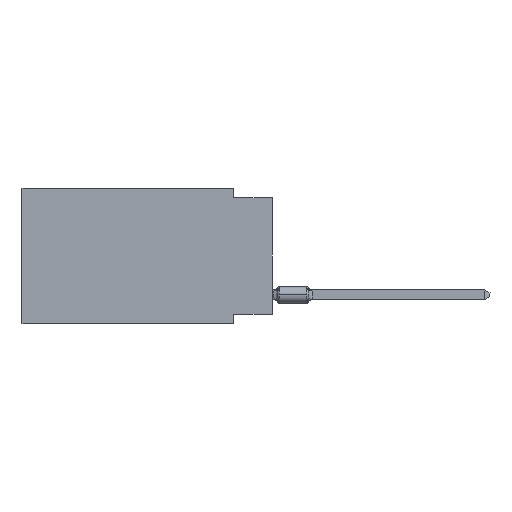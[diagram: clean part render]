
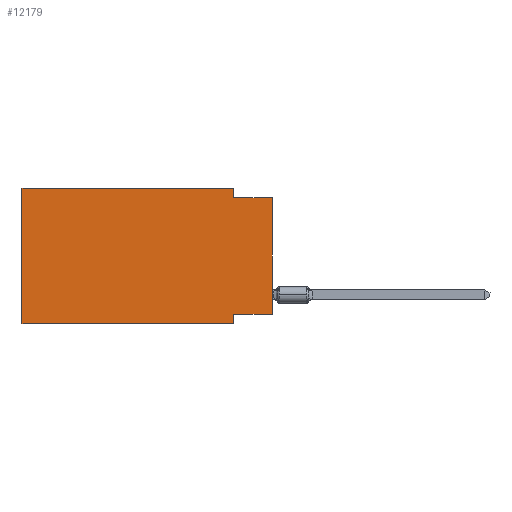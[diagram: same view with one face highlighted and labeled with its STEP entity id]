
A CAD part, left-side view. The second image highlights one B-rep face of the part: STEP entity #12179.
In plain terms, the highlighted planar face has unit normal (-1, 0, 0).
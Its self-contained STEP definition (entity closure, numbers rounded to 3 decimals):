
#191 = DIRECTION ( 'NONE',  ( 0., -1., 0. ) ) ;
#363 = EDGE_CURVE ( 'NONE', #18835, #9206, #13381, .T. ) ;
#1158 = VECTOR ( 'NONE', #7024, 1000. ) ;
#1394 = PLANE ( 'NONE',  #21384 ) ;
#1685 = DIRECTION ( 'NONE',  ( 0., 0., 1. ) ) ;
#1731 = CARTESIAN_POINT ( 'NONE',  ( 0., 0., -8.255 ) ) ;
#1751 = VECTOR ( 'NONE', #11459, 1000. ) ;
#1968 = DIRECTION ( 'NONE',  ( 0., 0., -1. ) ) ;
#2621 = ORIENTED_EDGE ( 'NONE', *, *, #363, .T. ) ;
#2857 = ORIENTED_EDGE ( 'NONE', *, *, #15554, .F. ) ;
#3054 = CARTESIAN_POINT ( 'NONE',  ( 0., 2.54, -8.89 ) ) ;
#4588 = EDGE_CURVE ( 'NONE', #18835, #18418, #22463, .T. ) ;
#4745 = CARTESIAN_POINT ( 'NONE',  ( 0., 16.383, -8.89 ) ) ;
#4921 = CARTESIAN_POINT ( 'NONE',  ( 0., 2.54, 0. ) ) ;
#6089 = VECTOR ( 'NONE', #29303, 1000. ) ;
#6251 = ORIENTED_EDGE ( 'NONE', *, *, #4588, .F. ) ;
#7024 = DIRECTION ( 'NONE',  ( 0., -1., 0. ) ) ;
#7233 = ORIENTED_EDGE ( 'NONE', *, *, #13359, .F. ) ;
#7501 = EDGE_CURVE ( 'NONE', #17132, #9206, #8265, .T. ) ;
#7999 = CARTESIAN_POINT ( 'NONE',  ( 0., 16.383, -8.89 ) ) ;
#8095 = CARTESIAN_POINT ( 'NONE',  ( 0., 0., -8.255 ) ) ;
#8265 = LINE ( 'NONE', #15932, #18362 ) ;
#8808 = EDGE_CURVE ( 'NONE', #25202, #20504, #13998, .T. ) ;
#9206 = VERTEX_POINT ( 'NONE', #28959 ) ;
#9609 = LINE ( 'NONE', #27790, #28229 ) ;
#11302 = ORIENTED_EDGE ( 'NONE', *, *, #7501, .F. ) ;
#11459 = DIRECTION ( 'NONE',  ( 0., 0., -1. ) ) ;
#12179 = ADVANCED_FACE ( 'NONE', ( #21865 ), #1394, .F. ) ;
#12879 = VECTOR ( 'NONE', #26718, 1000. ) ;
#13359 = EDGE_CURVE ( 'NONE', #18418, #23145, #26578, .T. ) ;
#13381 = LINE ( 'NONE', #24738, #22741 ) ;
#13714 = LINE ( 'NONE', #4745, #1158 ) ;
#13998 = LINE ( 'NONE', #23222, #14614 ) ;
#14471 = ORIENTED_EDGE ( 'NONE', *, *, #8808, .F. ) ;
#14550 = VERTEX_POINT ( 'NONE', #21872 ) ;
#14614 = VECTOR ( 'NONE', #27935, 1000. ) ;
#15401 = ORIENTED_EDGE ( 'NONE', *, *, #26850, .F. ) ;
#15554 = EDGE_CURVE ( 'NONE', #14550, #17132, #22824, .T. ) ;
#15932 = CARTESIAN_POINT ( 'NONE',  ( 0., 0., -0.635 ) ) ;
#17024 = CARTESIAN_POINT ( 'NONE',  ( 0., 2.54, -8.89 ) ) ;
#17132 = VERTEX_POINT ( 'NONE', #23230 ) ;
#17757 = DIRECTION ( 'NONE',  ( 1., 0., 0. ) ) ;
#18362 = VECTOR ( 'NONE', #25176, 1000. ) ;
#18418 = VERTEX_POINT ( 'NONE', #28716 ) ;
#18835 = VERTEX_POINT ( 'NONE', #1731 ) ;
#19474 = ORIENTED_EDGE ( 'NONE', *, *, #27826, .T. ) ;
#20504 = VERTEX_POINT ( 'NONE', #22627 ) ;
#21384 = AXIS2_PLACEMENT_3D ( 'NONE', #29724, #17757, #1968 ) ;
#21865 = FACE_OUTER_BOUND ( 'NONE', #28899, .T. ) ;
#21872 = CARTESIAN_POINT ( 'NONE',  ( 0., 2.54, 0. ) ) ;
#22463 = LINE ( 'NONE', #8095, #6089 ) ;
#22627 = CARTESIAN_POINT ( 'NONE',  ( 0., 16.383, 0. ) ) ;
#22741 = VECTOR ( 'NONE', #1685, 1000. ) ;
#22824 = LINE ( 'NONE', #4921, #1751 ) ;
#23145 = VERTEX_POINT ( 'NONE', #17024 ) ;
#23222 = CARTESIAN_POINT ( 'NONE',  ( 0., 16.383, 0. ) ) ;
#23230 = CARTESIAN_POINT ( 'NONE',  ( 0., 2.54, -0.635 ) ) ;
#24738 = CARTESIAN_POINT ( 'NONE',  ( 0., 0., 0. ) ) ;
#25176 = DIRECTION ( 'NONE',  ( 0., -1., 0. ) ) ;
#25202 = VERTEX_POINT ( 'NONE', #7999 ) ;
#26578 = LINE ( 'NONE', #3054, #12879 ) ;
#26718 = DIRECTION ( 'NONE',  ( 0., 0., -1. ) ) ;
#26850 = EDGE_CURVE ( 'NONE', #20504, #14550, #9609, .T. ) ;
#27790 = CARTESIAN_POINT ( 'NONE',  ( 0., 16.383, 0. ) ) ;
#27826 = EDGE_CURVE ( 'NONE', #25202, #23145, #13714, .T. ) ;
#27935 = DIRECTION ( 'NONE',  ( 0., 0., 1. ) ) ;
#28229 = VECTOR ( 'NONE', #191, 1000. ) ;
#28716 = CARTESIAN_POINT ( 'NONE',  ( 0., 2.54, -8.255 ) ) ;
#28899 = EDGE_LOOP ( 'NONE', ( #2621, #11302, #2857, #15401, #14471, #19474, #7233, #6251 ) ) ;
#28959 = CARTESIAN_POINT ( 'NONE',  ( 0., 0., -0.635 ) ) ;
#29303 = DIRECTION ( 'NONE',  ( 0., 1., 0. ) ) ;
#29724 = CARTESIAN_POINT ( 'NONE',  ( 0., 16.383, 0. ) ) ;
